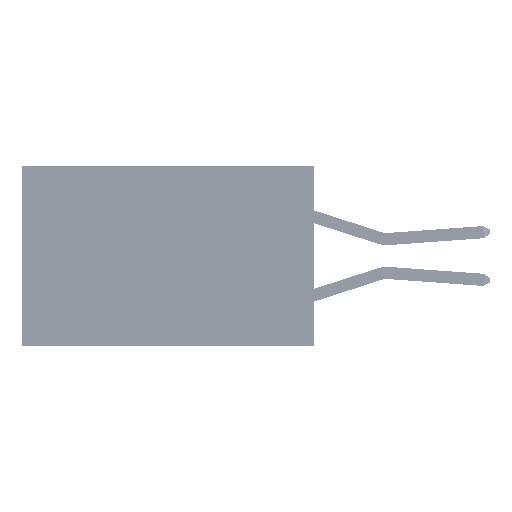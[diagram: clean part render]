
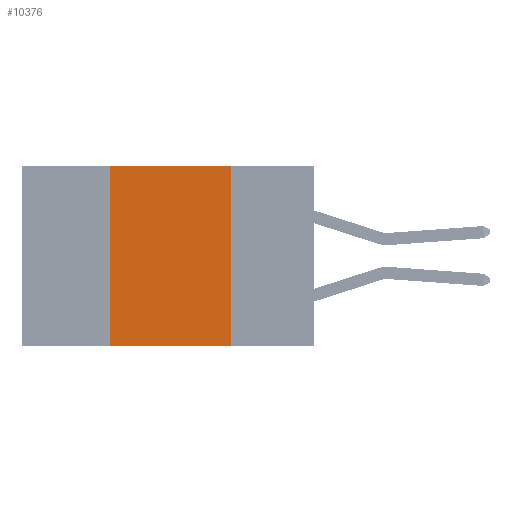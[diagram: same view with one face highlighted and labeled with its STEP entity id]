
A CAD part, left-side view. The second image highlights one B-rep face of the part: STEP entity #10376.
In plain terms, the highlighted planar face has unit normal (-1, 0, 0).
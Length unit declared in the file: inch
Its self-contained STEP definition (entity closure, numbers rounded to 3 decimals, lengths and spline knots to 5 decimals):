
#1761 = ORIENTED_EDGE ( 'NONE', *, *, #42403, .T. ) ;
#4816 = PLANE ( 'NONE',  #6542 ) ;
#6402 = CARTESIAN_POINT ( 'NONE',  ( 0., 0.17, 0. ) ) ;
#6542 = AXIS2_PLACEMENT_3D ( 'NONE', #30879, #15607, #19375 ) ;
#6735 = DIRECTION ( 'NONE',  ( 0., 0., -1. ) ) ;
#6927 = CARTESIAN_POINT ( 'NONE',  ( 0., 0.42, 0. ) ) ;
#7527 = LINE ( 'NONE', #23021, #45808 ) ;
#8352 = VECTOR ( 'NONE', #21933, 39.37008 ) ;
#9545 = LINE ( 'NONE', #6927, #8352 ) ;
#10365 = VERTEX_POINT ( 'NONE', #26900 ) ;
#10376 = ADVANCED_FACE ( 'NONE', ( #19826 ), #4816, .F. ) ;
#10466 = VECTOR ( 'NONE', #6735, 39.37008 ) ;
#11832 = DIRECTION ( 'NONE',  ( 0., -1., 0. ) ) ;
#15607 = DIRECTION ( 'NONE',  ( 1., 0., 0. ) ) ;
#18075 = VECTOR ( 'NONE', #37025, 39.37008 ) ;
#19375 = DIRECTION ( 'NONE',  ( 0., 0., -1. ) ) ;
#19826 = FACE_OUTER_BOUND ( 'NONE', #41010, .T. ) ;
#19922 = VERTEX_POINT ( 'NONE', #34035 ) ;
#21933 = DIRECTION ( 'NONE',  ( 0., 0., 1. ) ) ;
#23021 = CARTESIAN_POINT ( 'NONE',  ( 0., 0.6, 0. ) ) ;
#26900 = CARTESIAN_POINT ( 'NONE',  ( 0., 0.42, -0.37 ) ) ;
#28006 = VERTEX_POINT ( 'NONE', #46514 ) ;
#29848 = LINE ( 'NONE', #37194, #18075 ) ;
#30879 = CARTESIAN_POINT ( 'NONE',  ( 0., 0.6, 0. ) ) ;
#34035 = CARTESIAN_POINT ( 'NONE',  ( 0., 0.42, 0. ) ) ;
#34671 = ORIENTED_EDGE ( 'NONE', *, *, #35512, .F. ) ;
#35254 = EDGE_CURVE ( 'NONE', #45959, #28006, #35818, .T. ) ;
#35512 = EDGE_CURVE ( 'NONE', #19922, #45959, #7527, .T. ) ;
#35818 = LINE ( 'NONE', #6402, #10466 ) ;
#37025 = DIRECTION ( 'NONE',  ( 0., -1., 0. ) ) ;
#37194 = CARTESIAN_POINT ( 'NONE',  ( 0., 0.6, -0.37 ) ) ;
#40892 = ORIENTED_EDGE ( 'NONE', *, *, #35254, .F. ) ;
#41010 = EDGE_LOOP ( 'NONE', ( #40892, #34671, #44538, #1761 ) ) ;
#42403 = EDGE_CURVE ( 'NONE', #10365, #28006, #29848, .T. ) ;
#44538 = ORIENTED_EDGE ( 'NONE', *, *, #45178, .F. ) ;
#45178 = EDGE_CURVE ( 'NONE', #10365, #19922, #9545, .T. ) ;
#45808 = VECTOR ( 'NONE', #11832, 39.37008 ) ;
#45959 = VERTEX_POINT ( 'NONE', #48242 ) ;
#46514 = CARTESIAN_POINT ( 'NONE',  ( 0., 0.17, -0.37 ) ) ;
#48242 = CARTESIAN_POINT ( 'NONE',  ( 0., 0.17, 0. ) ) ;
